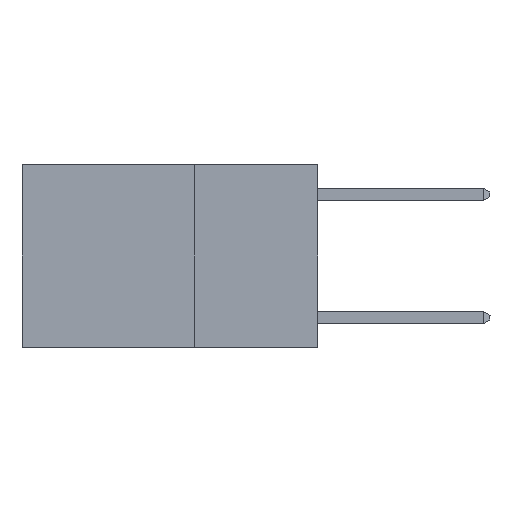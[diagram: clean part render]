
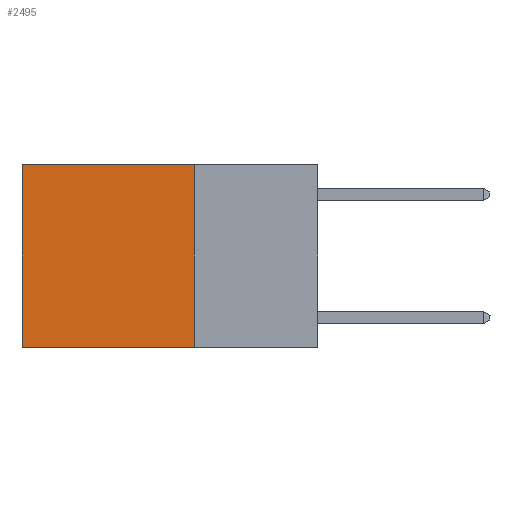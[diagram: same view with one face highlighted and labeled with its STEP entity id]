
A CAD part, left-side view. The second image highlights one B-rep face of the part: STEP entity #2495.
In plain terms, the highlighted planar face has unit normal (-1, 0, 0).
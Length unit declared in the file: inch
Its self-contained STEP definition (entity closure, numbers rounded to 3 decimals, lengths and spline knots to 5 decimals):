
#448 = DIRECTION ( 'NONE',  ( 0., 1., 0. ) ) ;
#524 = AXIS2_PLACEMENT_3D ( 'NONE', #9612, #3070, #10703 ) ;
#839 = ORIENTED_EDGE ( 'NONE', *, *, #10393, .T. ) ;
#1398 = LINE ( 'NONE', #6490, #12584 ) ;
#1536 = CARTESIAN_POINT ( 'NONE',  ( 0.2625, 0.25, 0. ) ) ;
#2495 = ADVANCED_FACE ( 'NONE', ( #8549 ), #13858, .F. ) ;
#2657 = CARTESIAN_POINT ( 'NONE',  ( 0.2625, 0.25, 0. ) ) ;
#3070 = DIRECTION ( 'NONE',  ( 1., 0., 0. ) ) ;
#3266 = VERTEX_POINT ( 'NONE', #4520 ) ;
#3299 = LINE ( 'NONE', #1536, #8744 ) ;
#3347 = ORIENTED_EDGE ( 'NONE', *, *, #3487, .T. ) ;
#3487 = EDGE_CURVE ( 'NONE', #9139, #6348, #12934, .T. ) ;
#4105 = CARTESIAN_POINT ( 'NONE',  ( 0.2625, 0.6, -0.37 ) ) ;
#4520 = CARTESIAN_POINT ( 'NONE',  ( 0.2625, 0.25, -0.37 ) ) ;
#5372 = CARTESIAN_POINT ( 'NONE',  ( 0.2625, 0.25, 0. ) ) ;
#6129 = EDGE_CURVE ( 'NONE', #13725, #3266, #13523, .T. ) ;
#6236 = ORIENTED_EDGE ( 'NONE', *, *, #12563, .F. ) ;
#6348 = VERTEX_POINT ( 'NONE', #4105 ) ;
#6490 = CARTESIAN_POINT ( 'NONE',  ( 0.2625, 0.25, -0.37 ) ) ;
#7152 = VECTOR ( 'NONE', #10320, 39.37008 ) ;
#8091 = VECTOR ( 'NONE', #9194, 39.37008 ) ;
#8549 = FACE_OUTER_BOUND ( 'NONE', #12072, .T. ) ;
#8686 = DIRECTION ( 'NONE',  ( 0., 1., 0. ) ) ;
#8744 = VECTOR ( 'NONE', #448, 39.37008 ) ;
#9139 = VERTEX_POINT ( 'NONE', #12369 ) ;
#9150 = ORIENTED_EDGE ( 'NONE', *, *, #6129, .F. ) ;
#9194 = DIRECTION ( 'NONE',  ( 0., 0., -1. ) ) ;
#9612 = CARTESIAN_POINT ( 'NONE',  ( 0.2625, 0.25, 0. ) ) ;
#10320 = DIRECTION ( 'NONE',  ( 0., 0., -1. ) ) ;
#10393 = EDGE_CURVE ( 'NONE', #13725, #9139, #3299, .T. ) ;
#10703 = DIRECTION ( 'NONE',  ( 0., 0., -1. ) ) ;
#12072 = EDGE_LOOP ( 'NONE', ( #3347, #6236, #9150, #839 ) ) ;
#12369 = CARTESIAN_POINT ( 'NONE',  ( 0.2625, 0.6, 0. ) ) ;
#12563 = EDGE_CURVE ( 'NONE', #3266, #6348, #1398, .T. ) ;
#12584 = VECTOR ( 'NONE', #8686, 39.37008 ) ;
#12934 = LINE ( 'NONE', #13467, #7152 ) ;
#13467 = CARTESIAN_POINT ( 'NONE',  ( 0.2625, 0.6, 0. ) ) ;
#13523 = LINE ( 'NONE', #2657, #8091 ) ;
#13725 = VERTEX_POINT ( 'NONE', #5372 ) ;
#13858 = PLANE ( 'NONE',  #524 ) ;
